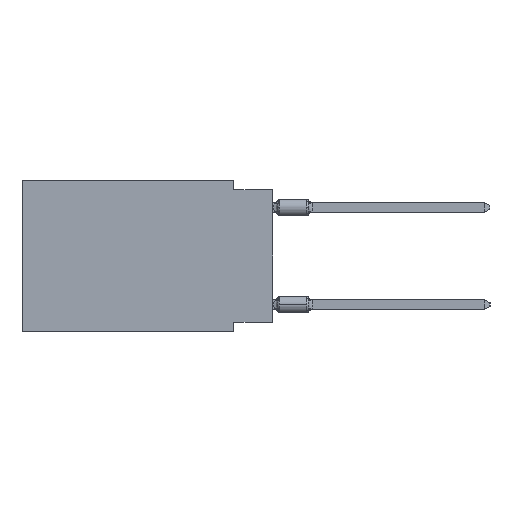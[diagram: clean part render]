
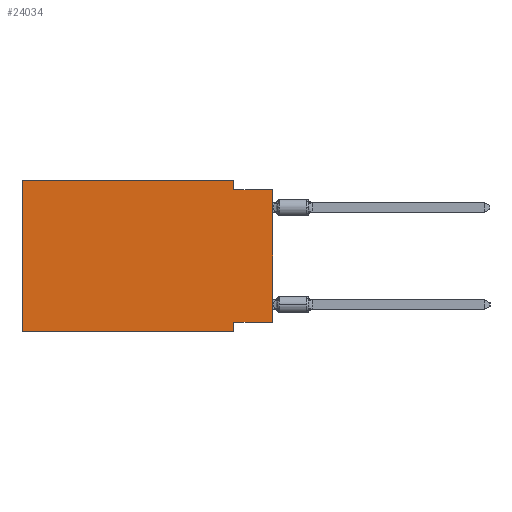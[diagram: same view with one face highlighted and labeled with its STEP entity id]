
A CAD part, left-side view. The second image highlights one B-rep face of the part: STEP entity #24034.
In plain terms, the highlighted planar face has unit normal (-1, 0, 0).
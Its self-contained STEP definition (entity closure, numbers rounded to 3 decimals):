
#1145 = CARTESIAN_POINT ( 'NONE',  ( 0., 0., -9.271 ) ) ;
#3923 = VERTEX_POINT ( 'NONE', #6100 ) ;
#4452 = LINE ( 'NONE', #1145, #36586 ) ;
#4761 = VERTEX_POINT ( 'NONE', #9264 ) ;
#5420 = EDGE_LOOP ( 'NONE', ( #29141, #23742, #39822, #40582, #42247, #28628, #7136, #5740 ) ) ;
#5740 = ORIENTED_EDGE ( 'NONE', *, *, #14791, .F. ) ;
#6001 = VERTEX_POINT ( 'NONE', #22620 ) ;
#6100 = CARTESIAN_POINT ( 'NONE',  ( 0., 2.54, 0. ) ) ;
#6373 = EDGE_CURVE ( 'NONE', #3923, #6001, #16101, .T. ) ;
#6625 = DIRECTION ( 'NONE',  ( 0., -1., 0. ) ) ;
#7136 = ORIENTED_EDGE ( 'NONE', *, *, #27965, .F. ) ;
#9264 = CARTESIAN_POINT ( 'NONE',  ( 0., 16.383, -9.906 ) ) ;
#9370 = PLANE ( 'NONE',  #24318 ) ;
#9600 = DIRECTION ( 'NONE',  ( 0., 0., -1. ) ) ;
#10399 = VERTEX_POINT ( 'NONE', #13757 ) ;
#11116 = VECTOR ( 'NONE', #18418, 1000. ) ;
#11351 = EDGE_CURVE ( 'NONE', #35443, #14266, #33717, .T. ) ;
#11592 = EDGE_CURVE ( 'NONE', #6001, #14266, #18204, .T. ) ;
#11988 = LINE ( 'NONE', #41905, #11116 ) ;
#12276 = CARTESIAN_POINT ( 'NONE',  ( 0., 16.383, 0. ) ) ;
#13757 = CARTESIAN_POINT ( 'NONE',  ( 0., 16.383, 0. ) ) ;
#13945 = CARTESIAN_POINT ( 'NONE',  ( 0., 0., -0.635 ) ) ;
#14266 = VERTEX_POINT ( 'NONE', #13945 ) ;
#14437 = DIRECTION ( 'NONE',  ( 0., 0., 1. ) ) ;
#14483 = VECTOR ( 'NONE', #14437, 1000. ) ;
#14791 = EDGE_CURVE ( 'NONE', #35443, #30969, #4452, .T. ) ;
#15566 = CARTESIAN_POINT ( 'NONE',  ( 0., 16.383, 0. ) ) ;
#16101 = LINE ( 'NONE', #37138, #42663 ) ;
#16207 = VERTEX_POINT ( 'NONE', #19715 ) ;
#16606 = LINE ( 'NONE', #36972, #23591 ) ;
#16955 = DIRECTION ( 'NONE',  ( 0., 0., -1. ) ) ;
#18204 = LINE ( 'NONE', #28162, #37850 ) ;
#18418 = DIRECTION ( 'NONE',  ( 0., 0., -1. ) ) ;
#18626 = CARTESIAN_POINT ( 'NONE',  ( 0., 0., -9.271 ) ) ;
#18841 = CARTESIAN_POINT ( 'NONE',  ( 0., 2.54, -9.271 ) ) ;
#19715 = CARTESIAN_POINT ( 'NONE',  ( 0., 2.54, -9.906 ) ) ;
#20612 = EDGE_CURVE ( 'NONE', #10399, #3923, #35100, .T. ) ;
#22620 = CARTESIAN_POINT ( 'NONE',  ( 0., 2.54, -0.635 ) ) ;
#22886 = DIRECTION ( 'NONE',  ( 1., 0., 0. ) ) ;
#23591 = VECTOR ( 'NONE', #6625, 1000. ) ;
#23742 = ORIENTED_EDGE ( 'NONE', *, *, #11592, .F. ) ;
#24034 = ADVANCED_FACE ( 'NONE', ( #26200 ), #9370, .F. ) ;
#24318 = AXIS2_PLACEMENT_3D ( 'NONE', #12276, #22886, #9600 ) ;
#24620 = CARTESIAN_POINT ( 'NONE',  ( 0., 0., 0. ) ) ;
#26200 = FACE_OUTER_BOUND ( 'NONE', #5420, .T. ) ;
#27965 = EDGE_CURVE ( 'NONE', #30969, #16207, #11988, .T. ) ;
#28158 = DIRECTION ( 'NONE',  ( 0., 1., 0. ) ) ;
#28162 = CARTESIAN_POINT ( 'NONE',  ( 0., 0., -0.635 ) ) ;
#28628 = ORIENTED_EDGE ( 'NONE', *, *, #43008, .T. ) ;
#29141 = ORIENTED_EDGE ( 'NONE', *, *, #11351, .T. ) ;
#30894 = CARTESIAN_POINT ( 'NONE',  ( 0., 16.383, 0. ) ) ;
#30969 = VERTEX_POINT ( 'NONE', #18841 ) ;
#31728 = DIRECTION ( 'NONE',  ( 0., -1., 0. ) ) ;
#32841 = LINE ( 'NONE', #15566, #40000 ) ;
#33717 = LINE ( 'NONE', #24620, #14483 ) ;
#35100 = LINE ( 'NONE', #30894, #38100 ) ;
#35443 = VERTEX_POINT ( 'NONE', #18626 ) ;
#36153 = DIRECTION ( 'NONE',  ( 0., 0., 1. ) ) ;
#36586 = VECTOR ( 'NONE', #28158, 1000. ) ;
#36972 = CARTESIAN_POINT ( 'NONE',  ( 0., 16.383, -9.906 ) ) ;
#37138 = CARTESIAN_POINT ( 'NONE',  ( 0., 2.54, 0. ) ) ;
#37850 = VECTOR ( 'NONE', #31728, 1000. ) ;
#38100 = VECTOR ( 'NONE', #41747, 1000. ) ;
#39822 = ORIENTED_EDGE ( 'NONE', *, *, #6373, .F. ) ;
#40000 = VECTOR ( 'NONE', #36153, 1000. ) ;
#40582 = ORIENTED_EDGE ( 'NONE', *, *, #20612, .F. ) ;
#40647 = EDGE_CURVE ( 'NONE', #4761, #10399, #32841, .T. ) ;
#41747 = DIRECTION ( 'NONE',  ( 0., -1., 0. ) ) ;
#41905 = CARTESIAN_POINT ( 'NONE',  ( 0., 2.54, -9.906 ) ) ;
#42247 = ORIENTED_EDGE ( 'NONE', *, *, #40647, .F. ) ;
#42663 = VECTOR ( 'NONE', #16955, 1000. ) ;
#43008 = EDGE_CURVE ( 'NONE', #4761, #16207, #16606, .T. ) ;
